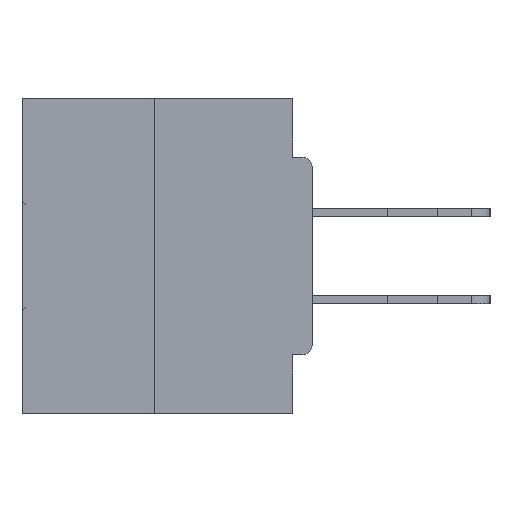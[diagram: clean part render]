
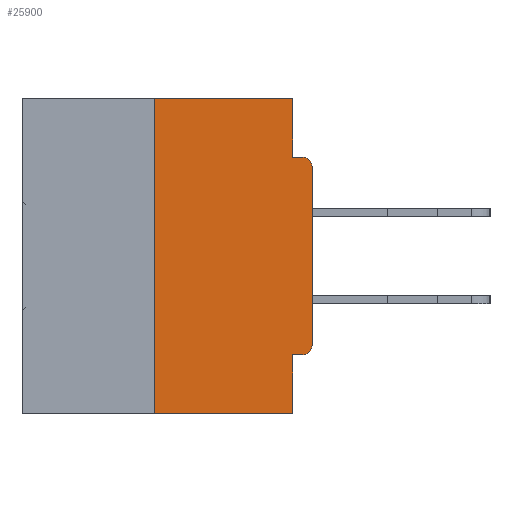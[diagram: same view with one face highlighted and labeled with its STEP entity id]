
A CAD part, left-side view. The second image highlights one B-rep face of the part: STEP entity #25900.
In plain terms, the highlighted planar face has unit normal (-1, 0, 0).
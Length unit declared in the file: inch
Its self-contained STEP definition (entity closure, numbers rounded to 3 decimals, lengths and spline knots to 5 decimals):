
#80 = CARTESIAN_POINT ( 'NONE',  ( 0., 0.031, 0. ) ) ;
#319 = LINE ( 'NONE', #20271, #19077 ) ;
#540 = ORIENTED_EDGE ( 'NONE', *, *, #16789, .T. ) ;
#1753 = CARTESIAN_POINT ( 'NONE',  ( 0., 0., -0.0935 ) ) ;
#2497 = DIRECTION ( 'NONE',  ( 0., -1., 0. ) ) ;
#2502 = EDGE_CURVE ( 'NONE', #42612, #41920, #15323, .T. ) ;
#2882 = CARTESIAN_POINT ( 'NONE',  ( 0., 0.031, 0. ) ) ;
#3211 = CARTESIAN_POINT ( 'NONE',  ( 0., 0.015, -0.1085 ) ) ;
#3359 = VECTOR ( 'NONE', #2497, 39.37008 ) ;
#4628 = ORIENTED_EDGE ( 'NONE', *, *, #7606, .T. ) ;
#4915 = CARTESIAN_POINT ( 'NONE',  ( 0., 0.015, -0.3915 ) ) ;
#5117 = VERTEX_POINT ( 'NONE', #34353 ) ;
#6074 = VERTEX_POINT ( 'NONE', #43279 ) ;
#6261 = EDGE_CURVE ( 'NONE', #36948, #29839, #8867, .T. ) ;
#7191 = ORIENTED_EDGE ( 'NONE', *, *, #22866, .F. ) ;
#7407 = DIRECTION ( 'NONE',  ( 0., 0., 1. ) ) ;
#7606 = EDGE_CURVE ( 'NONE', #19880, #33032, #25229, .T. ) ;
#8368 = VECTOR ( 'NONE', #12935, 39.37008 ) ;
#8867 = LINE ( 'NONE', #2882, #8368 ) ;
#8966 = CARTESIAN_POINT ( 'NONE',  ( 0., 0.031, -0.0935 ) ) ;
#9125 = DIRECTION ( 'NONE',  ( 0., -1., 0. ) ) ;
#9979 = EDGE_CURVE ( 'NONE', #29839, #33032, #21631, .T. ) ;
#10202 = EDGE_CURVE ( 'NONE', #5117, #41920, #26060, .T. ) ;
#10308 = VECTOR ( 'NONE', #42746, 39.37008 ) ;
#11352 = CIRCLE ( 'NONE', #28976, 0.015 ) ;
#12935 = DIRECTION ( 'NONE',  ( 0., 0., -1. ) ) ;
#13740 = CARTESIAN_POINT ( 'NONE',  ( 0., 0.031, -0.5 ) ) ;
#14329 = LINE ( 'NONE', #39135, #43591 ) ;
#15242 = CARTESIAN_POINT ( 'NONE',  ( 0., 0., -0.1085 ) ) ;
#15323 = LINE ( 'NONE', #38909, #10308 ) ;
#15912 = VERTEX_POINT ( 'NONE', #36568 ) ;
#16789 = EDGE_CURVE ( 'NONE', #26550, #19880, #14329, .T. ) ;
#16971 = LINE ( 'NONE', #20882, #36332 ) ;
#17725 = AXIS2_PLACEMENT_3D ( 'NONE', #29108, #29551, #18739 ) ;
#17973 = DIRECTION ( 'NONE',  ( 0., 0., 1. ) ) ;
#18739 = DIRECTION ( 'NONE',  ( 0., 0., -1. ) ) ;
#19077 = VECTOR ( 'NONE', #9125, 39.37008 ) ;
#19335 = DIRECTION ( 'NONE',  ( 0., -1., 0. ) ) ;
#19880 = VERTEX_POINT ( 'NONE', #15242 ) ;
#19941 = VECTOR ( 'NONE', #19335, 39.37008 ) ;
#20271 = CARTESIAN_POINT ( 'NONE',  ( 0., 0.46, 0. ) ) ;
#20791 = AXIS2_PLACEMENT_3D ( 'NONE', #3211, #45491, #27772 ) ;
#20882 = CARTESIAN_POINT ( 'NONE',  ( 0., 0.25, 0. ) ) ;
#21631 = LINE ( 'NONE', #1753, #19941 ) ;
#22075 = ORIENTED_EDGE ( 'NONE', *, *, #29997, .F. ) ;
#22866 = EDGE_CURVE ( 'NONE', #15912, #36948, #319, .T. ) ;
#23334 = ORIENTED_EDGE ( 'NONE', *, *, #6261, .F. ) ;
#23700 = CARTESIAN_POINT ( 'NONE',  ( 0., 0.46, -0.5 ) ) ;
#25229 = CIRCLE ( 'NONE', #20791, 0.015 ) ;
#25341 = VECTOR ( 'NONE', #32140, 39.37008 ) ;
#25900 = ADVANCED_FACE ( 'NONE', ( #43278 ), #36645, .F. ) ;
#26060 = LINE ( 'NONE', #23700, #3359 ) ;
#26124 = ORIENTED_EDGE ( 'NONE', *, *, #2502, .F. ) ;
#26550 = VERTEX_POINT ( 'NONE', #27253 ) ;
#27253 = CARTESIAN_POINT ( 'NONE',  ( 0., 0., -0.3915 ) ) ;
#27772 = DIRECTION ( 'NONE',  ( 0., 0., -1. ) ) ;
#28451 = CARTESIAN_POINT ( 'NONE',  ( 0., 0., -0.4065 ) ) ;
#28976 = AXIS2_PLACEMENT_3D ( 'NONE', #4915, #40733, #29663 ) ;
#29108 = CARTESIAN_POINT ( 'NONE',  ( 0., 0.46, 0. ) ) ;
#29551 = DIRECTION ( 'NONE',  ( 1., 0., 0. ) ) ;
#29663 = DIRECTION ( 'NONE',  ( 0., 0., -1. ) ) ;
#29839 = VERTEX_POINT ( 'NONE', #8966 ) ;
#29997 = EDGE_CURVE ( 'NONE', #5117, #15912, #16971, .T. ) ;
#30058 = EDGE_CURVE ( 'NONE', #6074, #42612, #42936, .T. ) ;
#30844 = ORIENTED_EDGE ( 'NONE', *, *, #38179, .T. ) ;
#30894 = ORIENTED_EDGE ( 'NONE', *, *, #30058, .F. ) ;
#31870 = CARTESIAN_POINT ( 'NONE',  ( 0., 0.015, -0.0935 ) ) ;
#32140 = DIRECTION ( 'NONE',  ( 0., 1., 0. ) ) ;
#33032 = VERTEX_POINT ( 'NONE', #31870 ) ;
#34353 = CARTESIAN_POINT ( 'NONE',  ( 0., 0.25, -0.5 ) ) ;
#36332 = VECTOR ( 'NONE', #7407, 39.37008 ) ;
#36568 = CARTESIAN_POINT ( 'NONE',  ( 0., 0.25, 0. ) ) ;
#36645 = PLANE ( 'NONE',  #17725 ) ;
#36948 = VERTEX_POINT ( 'NONE', #80 ) ;
#37448 = ORIENTED_EDGE ( 'NONE', *, *, #9979, .F. ) ;
#38179 = EDGE_CURVE ( 'NONE', #6074, #26550, #11352, .T. ) ;
#38909 = CARTESIAN_POINT ( 'NONE',  ( 0., 0.031, -0.5 ) ) ;
#39135 = CARTESIAN_POINT ( 'NONE',  ( 0., 0., 0. ) ) ;
#40733 = DIRECTION ( 'NONE',  ( -1., 0., 0. ) ) ;
#40975 = ORIENTED_EDGE ( 'NONE', *, *, #10202, .T. ) ;
#41524 = EDGE_LOOP ( 'NONE', ( #7191, #22075, #40975, #26124, #30894, #30844, #540, #4628, #37448, #23334 ) ) ;
#41920 = VERTEX_POINT ( 'NONE', #13740 ) ;
#42612 = VERTEX_POINT ( 'NONE', #43204 ) ;
#42746 = DIRECTION ( 'NONE',  ( 0., 0., -1. ) ) ;
#42936 = LINE ( 'NONE', #28451, #25341 ) ;
#43204 = CARTESIAN_POINT ( 'NONE',  ( 0., 0.031, -0.4065 ) ) ;
#43278 = FACE_OUTER_BOUND ( 'NONE', #41524, .T. ) ;
#43279 = CARTESIAN_POINT ( 'NONE',  ( 0., 0.015, -0.4065 ) ) ;
#43591 = VECTOR ( 'NONE', #17973, 39.37008 ) ;
#45491 = DIRECTION ( 'NONE',  ( -1., 0., 0. ) ) ;
